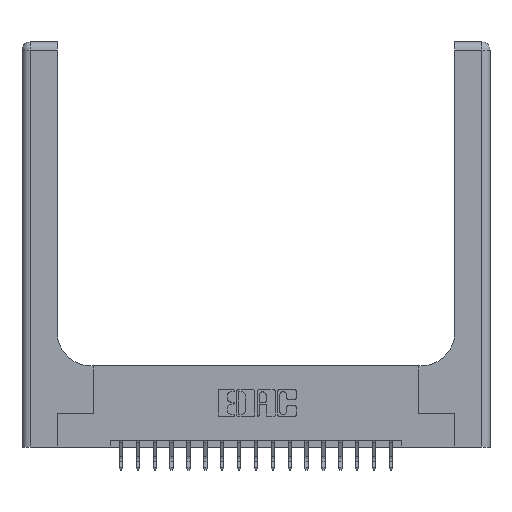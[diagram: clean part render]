
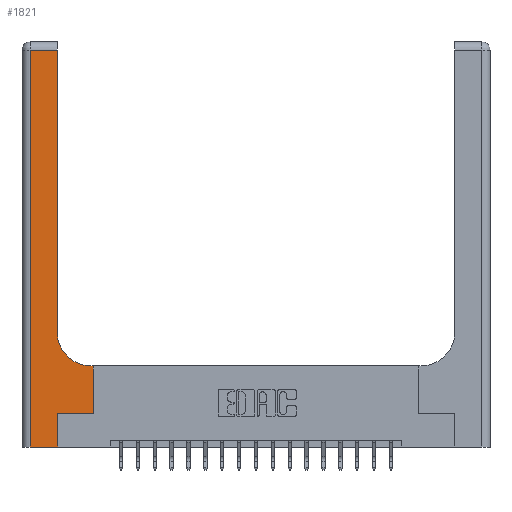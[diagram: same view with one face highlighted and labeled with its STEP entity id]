
A CAD part, top view. The second image highlights one B-rep face of the part: STEP entity #1821.
In plain terms, the highlighted planar face has unit normal (0, 0, 1).
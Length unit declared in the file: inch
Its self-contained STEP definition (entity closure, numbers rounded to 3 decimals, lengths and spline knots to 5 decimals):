
#157 = CARTESIAN_POINT ( 'NONE',  ( 0., 0., 0.37 ) ) ;
#306 = DIRECTION ( 'NONE',  ( -1., 0., 0. ) ) ;
#551 = AXIS2_PLACEMENT_3D ( 'NONE', #15559, #18777, #17353 ) ;
#714 = VECTOR ( 'NONE', #8995, 39.37008 ) ;
#736 = VERTEX_POINT ( 'NONE', #17014 ) ;
#825 = LINE ( 'NONE', #16401, #11398 ) ;
#1105 = VERTEX_POINT ( 'NONE', #12886 ) ;
#1383 = DIRECTION ( 'NONE',  ( 0., 1., 0. ) ) ;
#1821 = ADVANCED_FACE ( 'NONE', ( #5307 ), #13788, .F. ) ;
#2956 = EDGE_CURVE ( 'NONE', #15465, #16274, #14192, .T. ) ;
#3110 = CIRCLE ( 'NONE', #551, 0.25 ) ;
#3140 = LINE ( 'NONE', #16633, #714 ) ;
#3568 = VERTEX_POINT ( 'NONE', #19809 ) ;
#3750 = ORIENTED_EDGE ( 'NONE', *, *, #18280, .T. ) ;
#3899 = EDGE_CURVE ( 'NONE', #9121, #1105, #3110, .T. ) ;
#4098 = DIRECTION ( 'NONE',  ( 0., -1., 0. ) ) ;
#4237 = EDGE_CURVE ( 'NONE', #1105, #736, #5251, .T. ) ;
#4253 = CARTESIAN_POINT ( 'NONE',  ( 0.265, 0., 0.37 ) ) ;
#4405 = CARTESIAN_POINT ( 'NONE',  ( 0.528, 0.6, 0.37 ) ) ;
#4964 = LINE ( 'NONE', #10207, #6172 ) ;
#5111 = EDGE_LOOP ( 'NONE', ( #5792, #19069, #19276, #15655, #6942, #7579, #3750, #17395, #9983 ) ) ;
#5251 = LINE ( 'NONE', #8683, #7922 ) ;
#5307 = FACE_OUTER_BOUND ( 'NONE', #5111, .T. ) ;
#5381 = LINE ( 'NONE', #10172, #6594 ) ;
#5770 = DIRECTION ( 'NONE',  ( 0., 1., 0. ) ) ;
#5792 = ORIENTED_EDGE ( 'NONE', *, *, #4237, .T. ) ;
#5946 = CARTESIAN_POINT ( 'NONE',  ( 0.51, 0.6, 0.37 ) ) ;
#6043 = CARTESIAN_POINT ( 'NONE',  ( 0.265, 0.25, 0.37 ) ) ;
#6155 = DIRECTION ( 'NONE',  ( -1., 0., 0. ) ) ;
#6172 = VECTOR ( 'NONE', #4098, 39.37008 ) ;
#6292 = VERTEX_POINT ( 'NONE', #6043 ) ;
#6594 = VECTOR ( 'NONE', #11855, 39.37008 ) ;
#6942 = ORIENTED_EDGE ( 'NONE', *, *, #13736, .T. ) ;
#7194 = CARTESIAN_POINT ( 'NONE',  ( 0.528, 0.25, 0.37 ) ) ;
#7579 = ORIENTED_EDGE ( 'NONE', *, *, #16091, .T. ) ;
#7922 = VECTOR ( 'NONE', #5770, 39.37008 ) ;
#8683 = CARTESIAN_POINT ( 'NONE',  ( 0.26, 3., 0.37 ) ) ;
#8848 = LINE ( 'NONE', #14004, #9790 ) ;
#8995 = DIRECTION ( 'NONE',  ( 0., 1., 0. ) ) ;
#9069 = AXIS2_PLACEMENT_3D ( 'NONE', #11112, #9453, #6155 ) ;
#9121 = VERTEX_POINT ( 'NONE', #5946 ) ;
#9453 = DIRECTION ( 'NONE',  ( 0., 0., -1. ) ) ;
#9790 = VECTOR ( 'NONE', #306, 39.37008 ) ;
#9983 = ORIENTED_EDGE ( 'NONE', *, *, #3899, .T. ) ;
#10172 = CARTESIAN_POINT ( 'NONE',  ( 0.265, 0.25, 0.37 ) ) ;
#10207 = CARTESIAN_POINT ( 'NONE',  ( 0.06, 3., 0.37 ) ) ;
#10302 = EDGE_CURVE ( 'NONE', #736, #3568, #8848, .T. ) ;
#10370 = EDGE_CURVE ( 'NONE', #3568, #15465, #4964, .T. ) ;
#11094 = DIRECTION ( 'NONE',  ( 1., 0., 0. ) ) ;
#11112 = CARTESIAN_POINT ( 'NONE',  ( 0., 3., 0.37 ) ) ;
#11227 = VERTEX_POINT ( 'NONE', #4405 ) ;
#11398 = VECTOR ( 'NONE', #13448, 39.37008 ) ;
#11793 = EDGE_CURVE ( 'NONE', #11227, #9121, #825, .T. ) ;
#11855 = DIRECTION ( 'NONE',  ( 1., 0., 0. ) ) ;
#12886 = CARTESIAN_POINT ( 'NONE',  ( 0.26, 0.85, 0.37 ) ) ;
#13448 = DIRECTION ( 'NONE',  ( -1., 0., 0. ) ) ;
#13736 = EDGE_CURVE ( 'NONE', #16274, #6292, #14483, .T. ) ;
#13788 = PLANE ( 'NONE',  #9069 ) ;
#14004 = CARTESIAN_POINT ( 'NONE',  ( 0., 2.94, 0.37 ) ) ;
#14192 = LINE ( 'NONE', #157, #17073 ) ;
#14483 = LINE ( 'NONE', #18386, #17858 ) ;
#15338 = VERTEX_POINT ( 'NONE', #7194 ) ;
#15465 = VERTEX_POINT ( 'NONE', #19198 ) ;
#15559 = CARTESIAN_POINT ( 'NONE',  ( 0.51, 0.85, 0.37 ) ) ;
#15655 = ORIENTED_EDGE ( 'NONE', *, *, #2956, .T. ) ;
#16091 = EDGE_CURVE ( 'NONE', #6292, #15338, #5381, .T. ) ;
#16274 = VERTEX_POINT ( 'NONE', #4253 ) ;
#16401 = CARTESIAN_POINT ( 'NONE',  ( 0.26, 0.6, 0.37 ) ) ;
#16633 = CARTESIAN_POINT ( 'NONE',  ( 0.528, 0.25, 0.37 ) ) ;
#17014 = CARTESIAN_POINT ( 'NONE',  ( 0.26, 2.94, 0.37 ) ) ;
#17073 = VECTOR ( 'NONE', #11094, 39.37008 ) ;
#17353 = DIRECTION ( 'NONE',  ( 1., 0., 0. ) ) ;
#17395 = ORIENTED_EDGE ( 'NONE', *, *, #11793, .T. ) ;
#17858 = VECTOR ( 'NONE', #1383, 39.37008 ) ;
#18280 = EDGE_CURVE ( 'NONE', #15338, #11227, #3140, .T. ) ;
#18386 = CARTESIAN_POINT ( 'NONE',  ( 0.265, 0., 0.37 ) ) ;
#18777 = DIRECTION ( 'NONE',  ( 0., 0., -1. ) ) ;
#19069 = ORIENTED_EDGE ( 'NONE', *, *, #10302, .T. ) ;
#19198 = CARTESIAN_POINT ( 'NONE',  ( 0.06, 0., 0.37 ) ) ;
#19276 = ORIENTED_EDGE ( 'NONE', *, *, #10370, .T. ) ;
#19809 = CARTESIAN_POINT ( 'NONE',  ( 0.06, 2.94, 0.37 ) ) ;
